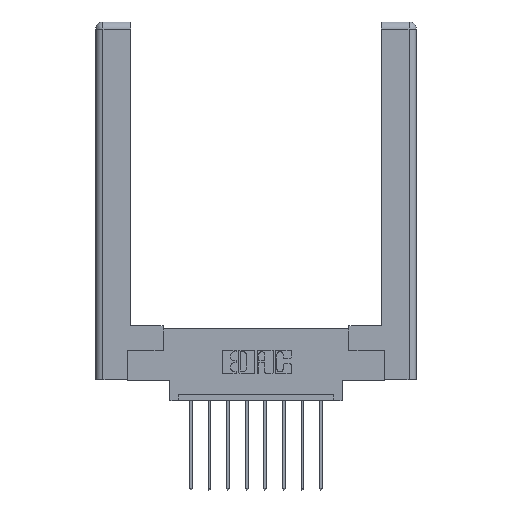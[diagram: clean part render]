
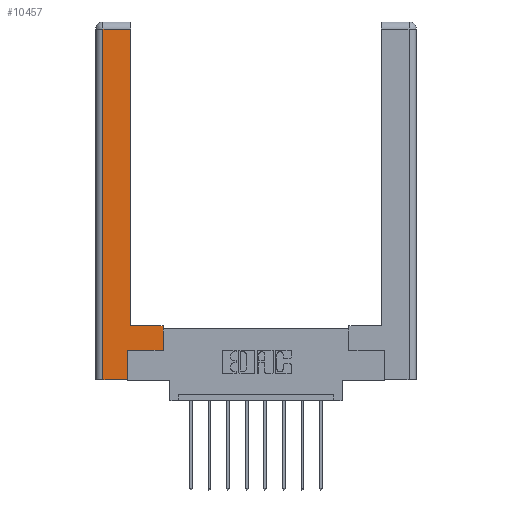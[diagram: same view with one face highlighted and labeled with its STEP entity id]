
A CAD part, top view. The second image highlights one B-rep face of the part: STEP entity #10457.
In plain terms, the highlighted planar face has unit normal (0, 0, 1).
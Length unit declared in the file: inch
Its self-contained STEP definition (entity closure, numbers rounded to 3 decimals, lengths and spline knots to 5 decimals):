
#471 = LINE ( 'NONE', #2722, #10473 ) ;
#606 = CARTESIAN_POINT ( 'NONE',  ( 0.565, 0.245, 0. ) ) ;
#614 = CARTESIAN_POINT ( 'NONE',  ( 0.565, 0.45, 0. ) ) ;
#744 = DIRECTION ( 'NONE',  ( 0., 1., 0. ) ) ;
#804 = CARTESIAN_POINT ( 'NONE',  ( 0.0615, 2.94, 0. ) ) ;
#1209 = VERTEX_POINT ( 'NONE', #5809 ) ;
#1267 = EDGE_CURVE ( 'NONE', #5621, #7390, #9807, .T. ) ;
#1406 = CARTESIAN_POINT ( 'NONE',  ( 0.295, 0.45, 0. ) ) ;
#1539 = EDGE_CURVE ( 'NONE', #7168, #6109, #13119, .T. ) ;
#1564 = DIRECTION ( 'NONE',  ( -1., 0., 0. ) ) ;
#1694 = ORIENTED_EDGE ( 'NONE', *, *, #7642, .T. ) ;
#2238 = EDGE_LOOP ( 'NONE', ( #9036, #12793, #8247, #1694, #6063, #7267, #4585, #4190 ) ) ;
#2722 = CARTESIAN_POINT ( 'NONE',  ( 0.265, 0., 0. ) ) ;
#2872 = DIRECTION ( 'NONE',  ( 0., 1., 0. ) ) ;
#3002 = CARTESIAN_POINT ( 'NONE',  ( 0.565, 0.245, 0. ) ) ;
#3749 = FACE_OUTER_BOUND ( 'NONE', #2238, .T. ) ;
#3809 = CARTESIAN_POINT ( 'NONE',  ( 0.295, 3., 0. ) ) ;
#3886 = CARTESIAN_POINT ( 'NONE',  ( 0.0615, 0., 0. ) ) ;
#4190 = ORIENTED_EDGE ( 'NONE', *, *, #7946, .T. ) ;
#4349 = EDGE_CURVE ( 'NONE', #12361, #10119, #6245, .T. ) ;
#4585 = ORIENTED_EDGE ( 'NONE', *, *, #4349, .T. ) ;
#4735 = VERTEX_POINT ( 'NONE', #12605 ) ;
#5621 = VERTEX_POINT ( 'NONE', #8186 ) ;
#5809 = CARTESIAN_POINT ( 'NONE',  ( 0.295, 0.45, 0. ) ) ;
#5917 = VECTOR ( 'NONE', #744, 39.37008 ) ;
#6063 = ORIENTED_EDGE ( 'NONE', *, *, #1539, .T. ) ;
#6109 = VERTEX_POINT ( 'NONE', #11907 ) ;
#6127 = VECTOR ( 'NONE', #10961, 39.37008 ) ;
#6245 = LINE ( 'NONE', #614, #5917 ) ;
#6308 = VECTOR ( 'NONE', #12798, 39.37008 ) ;
#6640 = DIRECTION ( 'NONE',  ( -1., 0., 0. ) ) ;
#6864 = EDGE_CURVE ( 'NONE', #7390, #4735, #11925, .T. ) ;
#7076 = LINE ( 'NONE', #3809, #6127 ) ;
#7168 = VERTEX_POINT ( 'NONE', #12341 ) ;
#7267 = ORIENTED_EDGE ( 'NONE', *, *, #10104, .T. ) ;
#7272 = VECTOR ( 'NONE', #1564, 39.37008 ) ;
#7390 = VERTEX_POINT ( 'NONE', #804 ) ;
#7642 = EDGE_CURVE ( 'NONE', #4735, #7168, #471, .T. ) ;
#7644 = PLANE ( 'NONE',  #12521 ) ;
#7695 = VECTOR ( 'NONE', #2872, 39.37008 ) ;
#7945 = CARTESIAN_POINT ( 'NONE',  ( 0.565, 0.45, 0. ) ) ;
#7946 = EDGE_CURVE ( 'NONE', #10119, #1209, #11579, .T. ) ;
#8186 = CARTESIAN_POINT ( 'NONE',  ( 0.295, 2.94, 0. ) ) ;
#8247 = ORIENTED_EDGE ( 'NONE', *, *, #6864, .T. ) ;
#8591 = VECTOR ( 'NONE', #11027, 39.37008 ) ;
#8838 = DIRECTION ( 'NONE',  ( 1., 0., 0. ) ) ;
#8840 = VECTOR ( 'NONE', #8928, 39.37008 ) ;
#8845 = LINE ( 'NONE', #606, #6308 ) ;
#8928 = DIRECTION ( 'NONE',  ( -1., 0., 0. ) ) ;
#8954 = CARTESIAN_POINT ( 'NONE',  ( 0.265, 0.245, 0. ) ) ;
#9036 = ORIENTED_EDGE ( 'NONE', *, *, #11455, .T. ) ;
#9675 = CARTESIAN_POINT ( 'NONE',  ( 0., 0., 0. ) ) ;
#9807 = LINE ( 'NONE', #10896, #8840 ) ;
#10104 = EDGE_CURVE ( 'NONE', #6109, #12361, #8845, .T. ) ;
#10119 = VERTEX_POINT ( 'NONE', #7945 ) ;
#10457 = ADVANCED_FACE ( 'NONE', ( #3749 ), #7644, .F. ) ;
#10473 = VECTOR ( 'NONE', #8838, 39.37008 ) ;
#10896 = CARTESIAN_POINT ( 'NONE',  ( 0.0615, 2.94, 0. ) ) ;
#10961 = DIRECTION ( 'NONE',  ( 0., 1., 0. ) ) ;
#11027 = DIRECTION ( 'NONE',  ( 0., -1., 0. ) ) ;
#11455 = EDGE_CURVE ( 'NONE', #1209, #5621, #7076, .T. ) ;
#11579 = LINE ( 'NONE', #1406, #7272 ) ;
#11907 = CARTESIAN_POINT ( 'NONE',  ( 0.265, 0.245, 0. ) ) ;
#11925 = LINE ( 'NONE', #3886, #8591 ) ;
#12341 = CARTESIAN_POINT ( 'NONE',  ( 0.265, 0., 0. ) ) ;
#12361 = VERTEX_POINT ( 'NONE', #3002 ) ;
#12521 = AXIS2_PLACEMENT_3D ( 'NONE', #9675, #12815, #6640 ) ;
#12605 = CARTESIAN_POINT ( 'NONE',  ( 0.0615, 0., 0. ) ) ;
#12793 = ORIENTED_EDGE ( 'NONE', *, *, #1267, .T. ) ;
#12798 = DIRECTION ( 'NONE',  ( 1., 0., 0. ) ) ;
#12815 = DIRECTION ( 'NONE',  ( 0., 0., -1. ) ) ;
#13119 = LINE ( 'NONE', #8954, #7695 ) ;
